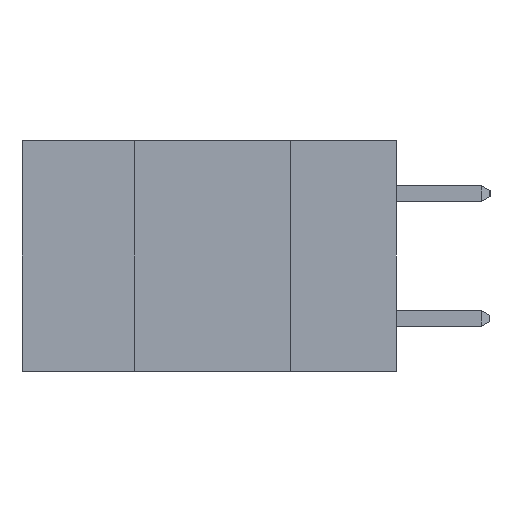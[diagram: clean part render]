
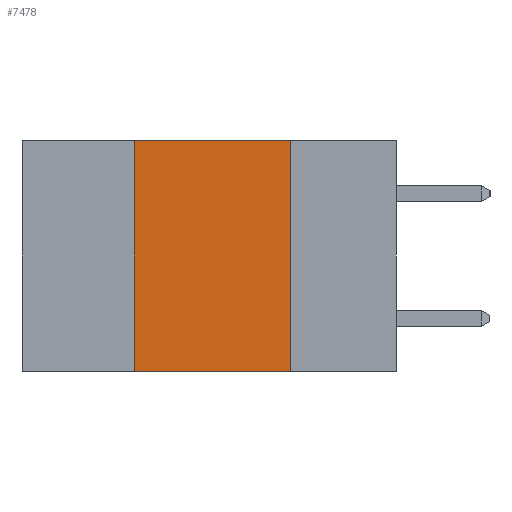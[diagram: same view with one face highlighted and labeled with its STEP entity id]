
A CAD part, left-side view. The second image highlights one B-rep face of the part: STEP entity #7478.
In plain terms, the highlighted planar face has unit normal (-1, 0, 0).
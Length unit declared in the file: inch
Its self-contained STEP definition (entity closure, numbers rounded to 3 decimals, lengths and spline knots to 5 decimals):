
#358 = VECTOR ( 'NONE', #12177, 39.37008 ) ;
#1141 = CARTESIAN_POINT ( 'NONE',  ( 0., 0.42, -0.37 ) ) ;
#1345 = DIRECTION ( 'NONE',  ( 0., 0., -1. ) ) ;
#1501 = ORIENTED_EDGE ( 'NONE', *, *, #18154, .F. ) ;
#2211 = LINE ( 'NONE', #3734, #18906 ) ;
#2755 = PLANE ( 'NONE',  #14434 ) ;
#2938 = ORIENTED_EDGE ( 'NONE', *, *, #14597, .T. ) ;
#3734 = CARTESIAN_POINT ( 'NONE',  ( 0., 0.17, -0.37 ) ) ;
#3887 = VERTEX_POINT ( 'NONE', #14689 ) ;
#4378 = LINE ( 'NONE', #13971, #358 ) ;
#4898 = LINE ( 'NONE', #6232, #8248 ) ;
#5435 = EDGE_CURVE ( 'NONE', #3887, #8742, #13880, .T. ) ;
#6232 = CARTESIAN_POINT ( 'NONE',  ( 0., 0.42, -0.37 ) ) ;
#7478 = ADVANCED_FACE ( 'NONE', ( #17025 ), #2755, .F. ) ;
#8022 = DIRECTION ( 'NONE',  ( 0., -1., 0. ) ) ;
#8248 = VECTOR ( 'NONE', #15521, 39.37008 ) ;
#8556 = CARTESIAN_POINT ( 'NONE',  ( 0., 0.17, 0. ) ) ;
#8701 = VERTEX_POINT ( 'NONE', #14694 ) ;
#8742 = VERTEX_POINT ( 'NONE', #8556 ) ;
#10768 = CARTESIAN_POINT ( 'NONE',  ( 0., 0.6, 0. ) ) ;
#12177 = DIRECTION ( 'NONE',  ( 0., -1., 0. ) ) ;
#12369 = DIRECTION ( 'NONE',  ( 1., 0., 0. ) ) ;
#13115 = VERTEX_POINT ( 'NONE', #1141 ) ;
#13597 = EDGE_CURVE ( 'NONE', #8742, #8701, #2211, .T. ) ;
#13880 = LINE ( 'NONE', #18534, #15039 ) ;
#13971 = CARTESIAN_POINT ( 'NONE',  ( 0., 0.6, -0.37 ) ) ;
#14434 = AXIS2_PLACEMENT_3D ( 'NONE', #10768, #12369, #1345 ) ;
#14597 = EDGE_CURVE ( 'NONE', #13115, #8701, #4378, .T. ) ;
#14689 = CARTESIAN_POINT ( 'NONE',  ( 0., 0.42, 0. ) ) ;
#14694 = CARTESIAN_POINT ( 'NONE',  ( 0., 0.17, -0.37 ) ) ;
#14806 = EDGE_LOOP ( 'NONE', ( #17950, #18270, #1501, #2938 ) ) ;
#15039 = VECTOR ( 'NONE', #8022, 39.37008 ) ;
#15521 = DIRECTION ( 'NONE',  ( 0., 0., 1. ) ) ;
#16390 = DIRECTION ( 'NONE',  ( 0., 0., -1. ) ) ;
#17025 = FACE_OUTER_BOUND ( 'NONE', #14806, .T. ) ;
#17950 = ORIENTED_EDGE ( 'NONE', *, *, #13597, .F. ) ;
#18154 = EDGE_CURVE ( 'NONE', #13115, #3887, #4898, .T. ) ;
#18270 = ORIENTED_EDGE ( 'NONE', *, *, #5435, .F. ) ;
#18534 = CARTESIAN_POINT ( 'NONE',  ( 0., 0.6, 0. ) ) ;
#18906 = VECTOR ( 'NONE', #16390, 39.37008 ) ;
